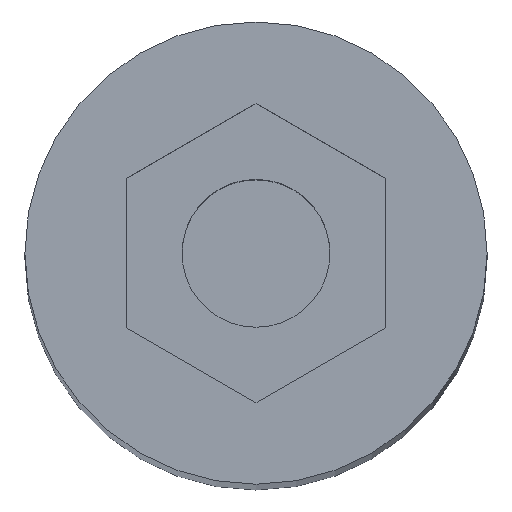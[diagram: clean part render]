
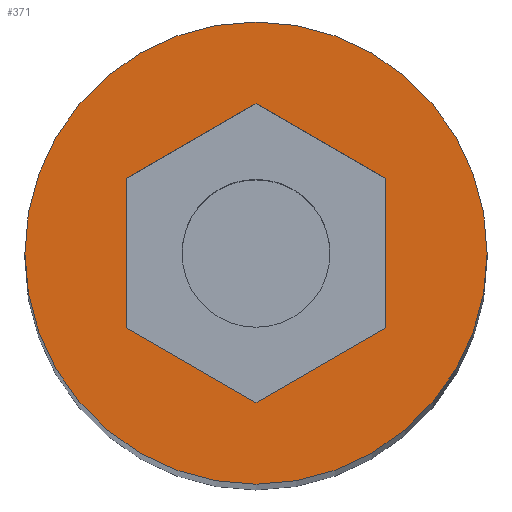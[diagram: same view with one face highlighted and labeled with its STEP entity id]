
A CAD part, top view. The second image highlights one B-rep face of the part: STEP entity #371.
In plain terms, the highlighted planar face has unit normal (0, 0, 1).
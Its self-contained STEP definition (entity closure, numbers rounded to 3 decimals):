
#3 = CARTESIAN_POINT ( 'NONE',  ( 3.75, 0., 53.75 ) ) ;
#6 = CARTESIAN_POINT ( 'NONE',  ( 0., 0., 53.75 ) ) ;
#13 = CARTESIAN_POINT ( 'NONE',  ( 0., 0., 53.75 ) ) ;
#14 = CARTESIAN_POINT ( 'NONE',  ( 0., 2.427, 53.75 ) ) ;
#15 = AXIS2_PLACEMENT_3D ( 'NONE', #26, #163, #40 ) ;
#16 = DIRECTION ( 'NONE',  ( 0.866, 0.5, 0. ) ) ;
#17 = AXIS2_PLACEMENT_3D ( 'NONE', #6, #389, #248 ) ;
#19 = CARTESIAN_POINT ( 'NONE',  ( 0., 2.427, 53.75 ) ) ;
#26 = CARTESIAN_POINT ( 'NONE',  ( 0., 0., 53.75 ) ) ;
#28 = DIRECTION ( 'NONE',  ( 1., 0., 0. ) ) ;
#36 = AXIS2_PLACEMENT_3D ( 'NONE', #13, #122, #28 ) ;
#37 = CARTESIAN_POINT ( 'NONE',  ( -2.102, -1.213, 53.75 ) ) ;
#40 = DIRECTION ( 'NONE',  ( 1., 0., 0. ) ) ;
#43 = CARTESIAN_POINT ( 'NONE',  ( 2.102, 1.213, 53.75 ) ) ;
#46 = CARTESIAN_POINT ( 'NONE',  ( 2.102, 1.213, 53.75 ) ) ;
#57 = DIRECTION ( 'NONE',  ( -0.866, 0.5, 0. ) ) ;
#70 = PLANE ( 'NONE',  #17 ) ;
#74 = DIRECTION ( 'NONE',  ( 0., -1., 0. ) ) ;
#106 = CARTESIAN_POINT ( 'NONE',  ( 0., -2.427, 53.75 ) ) ;
#122 = DIRECTION ( 'NONE',  ( 0., 0., 1. ) ) ;
#130 = DIRECTION ( 'NONE',  ( 0.866, -0.5, 0. ) ) ;
#150 = CARTESIAN_POINT ( 'NONE',  ( 2.102, -1.213, 53.75 ) ) ;
#154 = DIRECTION ( 'NONE',  ( 0., 1., 0. ) ) ;
#163 = DIRECTION ( 'NONE',  ( 0., 0., 1. ) ) ;
#170 = DIRECTION ( 'NONE',  ( -0.866, -0.5, 0. ) ) ;
#172 = CARTESIAN_POINT ( 'NONE',  ( -2.102, 1.213, 53.75 ) ) ;
#177 = VECTOR ( 'NONE', #170, 1000. ) ;
#180 = VECTOR ( 'NONE', #74, 1000. ) ;
#183 = LINE ( 'NONE', #233, #180 ) ;
#185 = LINE ( 'NONE', #14, #177 ) ;
#186 = VECTOR ( 'NONE', #130, 1000. ) ;
#188 = LINE ( 'NONE', #43, #191 ) ;
#190 = VECTOR ( 'NONE', #16, 1000. ) ;
#191 = VECTOR ( 'NONE', #57, 1000. ) ;
#193 = LINE ( 'NONE', #340, #190 ) ;
#194 = VECTOR ( 'NONE', #154, 1000. ) ;
#199 = LINE ( 'NONE', #37, #186 ) ;
#201 = CARTESIAN_POINT ( 'NONE',  ( 2.102, -1.213, 53.75 ) ) ;
#206 = LINE ( 'NONE', #201, #194 ) ;
#208 = CIRCLE ( 'NONE', #15, 3.75 ) ;
#217 = FACE_OUTER_BOUND ( 'NONE', #275, .T. ) ;
#221 = FACE_BOUND ( 'NONE', #341, .T. ) ;
#231 = CARTESIAN_POINT ( 'NONE',  ( -3.75, 0., 53.75 ) ) ;
#233 = CARTESIAN_POINT ( 'NONE',  ( -2.102, 1.213, 53.75 ) ) ;
#243 = CIRCLE ( 'NONE', #36, 3.75 ) ;
#248 = DIRECTION ( 'NONE',  ( 1., 0., 0. ) ) ;
#262 = ORIENTED_EDGE ( 'NONE', *, *, #414, .F. ) ;
#263 = ORIENTED_EDGE ( 'NONE', *, *, #415, .F. ) ;
#269 = ORIENTED_EDGE ( 'NONE', *, *, #380, .T. ) ;
#270 = ORIENTED_EDGE ( 'NONE', *, *, #359, .T. ) ;
#275 = EDGE_LOOP ( 'NONE', ( #269, #270 ) ) ;
#322 = VERTEX_POINT ( 'NONE', #19 ) ;
#340 = CARTESIAN_POINT ( 'NONE',  ( 0., -2.427, 53.75 ) ) ;
#341 = EDGE_LOOP ( 'NONE', ( #388, #392, #385, #390, #262, #263 ) ) ;
#359 = EDGE_CURVE ( 'NONE', #435, #431, #243, .T. ) ;
#371 = ADVANCED_FACE ( 'NONE', ( #221, #217 ), #70, .T. ) ;
#380 = EDGE_CURVE ( 'NONE', #431, #435, #208, .T. ) ;
#385 = ORIENTED_EDGE ( 'NONE', *, *, #402, .F. ) ;
#388 = ORIENTED_EDGE ( 'NONE', *, *, #393, .F. ) ;
#389 = DIRECTION ( 'NONE',  ( 0., 0., 1. ) ) ;
#390 = ORIENTED_EDGE ( 'NONE', *, *, #410, .F. ) ;
#392 = ORIENTED_EDGE ( 'NONE', *, *, #400, .F. ) ;
#393 = EDGE_CURVE ( 'NONE', #458, #408, #206, .T. ) ;
#397 = CARTESIAN_POINT ( 'NONE',  ( -2.102, -1.213, 53.75 ) ) ;
#400 = EDGE_CURVE ( 'NONE', #424, #458, #193, .T. ) ;
#402 = EDGE_CURVE ( 'NONE', #421, #424, #199, .T. ) ;
#408 = VERTEX_POINT ( 'NONE', #46 ) ;
#410 = EDGE_CURVE ( 'NONE', #441, #421, #183, .T. ) ;
#414 = EDGE_CURVE ( 'NONE', #322, #441, #185, .T. ) ;
#415 = EDGE_CURVE ( 'NONE', #408, #322, #188, .T. ) ;
#421 = VERTEX_POINT ( 'NONE', #397 ) ;
#424 = VERTEX_POINT ( 'NONE', #106 ) ;
#431 = VERTEX_POINT ( 'NONE', #231 ) ;
#435 = VERTEX_POINT ( 'NONE', #3 ) ;
#441 = VERTEX_POINT ( 'NONE', #172 ) ;
#458 = VERTEX_POINT ( 'NONE', #150 ) ;
